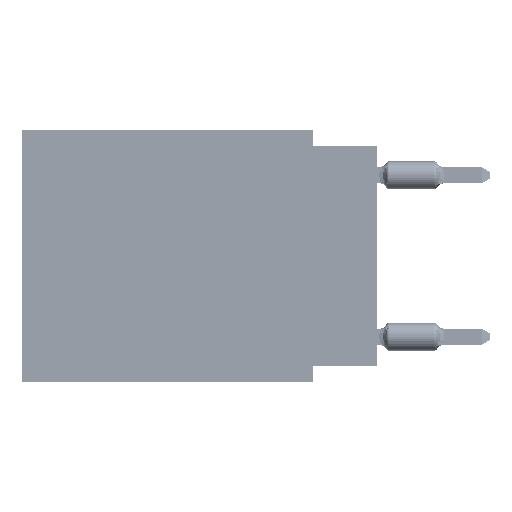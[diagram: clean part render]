
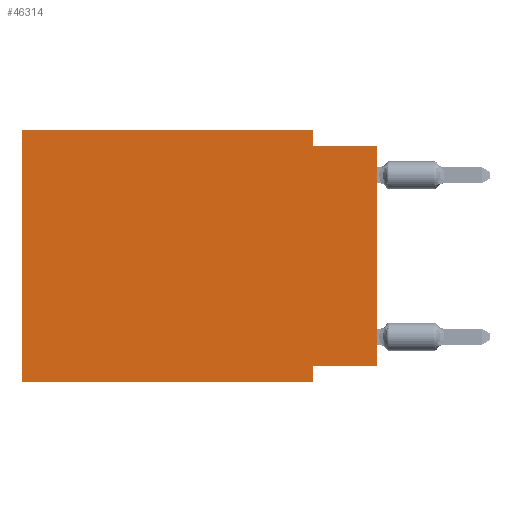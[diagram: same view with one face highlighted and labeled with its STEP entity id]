
A CAD part, left-side view. The second image highlights one B-rep face of the part: STEP entity #46314.
In plain terms, the highlighted planar face has unit normal (-1, 0, 0).
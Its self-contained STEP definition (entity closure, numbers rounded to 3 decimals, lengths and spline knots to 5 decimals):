
#1452 = DIRECTION ( 'NONE',  ( 0., 1., 0. ) ) ;
#3383 = LINE ( 'NONE', #30743, #34249 ) ;
#4033 = LINE ( 'NONE', #73590, #63360 ) ;
#4944 = DIRECTION ( 'NONE',  ( 0., 0., -1. ) ) ;
#5041 = CARTESIAN_POINT ( 'NONE',  ( 0., 0.1, -0.365 ) ) ;
#6688 = VERTEX_POINT ( 'NONE', #30432 ) ;
#10154 = CARTESIAN_POINT ( 'NONE',  ( 0., 0., -0.025 ) ) ;
#11012 = VERTEX_POINT ( 'NONE', #65334 ) ;
#11158 = EDGE_CURVE ( 'NONE', #77506, #37980, #19530, .T. ) ;
#14460 = LINE ( 'NONE', #21627, #53248 ) ;
#15268 = CARTESIAN_POINT ( 'NONE',  ( 0., 0.55, -0.39 ) ) ;
#15789 = EDGE_LOOP ( 'NONE', ( #80450, #38972, #65333, #28414, #53009, #39994, #20164, #63234 ) ) ;
#15989 = DIRECTION ( 'NONE',  ( 0., 0., -1. ) ) ;
#16854 = LINE ( 'NONE', #22697, #59315 ) ;
#19530 = LINE ( 'NONE', #46908, #31091 ) ;
#20164 = ORIENTED_EDGE ( 'NONE', *, *, #22081, .F. ) ;
#21627 = CARTESIAN_POINT ( 'NONE',  ( 0., 0., -0.365 ) ) ;
#22081 = EDGE_CURVE ( 'NONE', #63224, #22983, #4033, .T. ) ;
#22697 = CARTESIAN_POINT ( 'NONE',  ( 0., 0.1, 0. ) ) ;
#22983 = VERTEX_POINT ( 'NONE', #27564 ) ;
#25158 = EDGE_CURVE ( 'NONE', #77506, #22983, #75802, .T. ) ;
#27564 = CARTESIAN_POINT ( 'NONE',  ( 0., 0.1, -0.39 ) ) ;
#28414 = ORIENTED_EDGE ( 'NONE', *, *, #62690, .F. ) ;
#28687 = DIRECTION ( 'NONE',  ( 0., -1., 0. ) ) ;
#30432 = CARTESIAN_POINT ( 'NONE',  ( 0., 0.1, -0.025 ) ) ;
#30743 = CARTESIAN_POINT ( 'NONE',  ( 0., 0.55, 0. ) ) ;
#31091 = VECTOR ( 'NONE', #52775, 39.37008 ) ;
#32036 = CARTESIAN_POINT ( 'NONE',  ( 0., 0., 0. ) ) ;
#32081 = DIRECTION ( 'NONE',  ( 0., -1., 0. ) ) ;
#34249 = VECTOR ( 'NONE', #32081, 39.37008 ) ;
#37980 = VERTEX_POINT ( 'NONE', #38808 ) ;
#38755 = LINE ( 'NONE', #32036, #80571 ) ;
#38808 = CARTESIAN_POINT ( 'NONE',  ( 0., 0.55, 0. ) ) ;
#38972 = ORIENTED_EDGE ( 'NONE', *, *, #40703, .F. ) ;
#39994 = ORIENTED_EDGE ( 'NONE', *, *, #25158, .T. ) ;
#40703 = EDGE_CURVE ( 'NONE', #6688, #11012, #72194, .T. ) ;
#41505 = VERTEX_POINT ( 'NONE', #70709 ) ;
#46314 = ADVANCED_FACE ( 'NONE', ( #53259 ), #80597, .F. ) ;
#46908 = CARTESIAN_POINT ( 'NONE',  ( 0., 0.55, 0. ) ) ;
#48878 = EDGE_CURVE ( 'NONE', #67339, #11012, #38755, .T. ) ;
#48914 = CARTESIAN_POINT ( 'NONE',  ( 0., 0.55, -0.39 ) ) ;
#49573 = VECTOR ( 'NONE', #28687, 39.37008 ) ;
#49673 = DIRECTION ( 'NONE',  ( 0., -1., 0. ) ) ;
#50067 = CARTESIAN_POINT ( 'NONE',  ( 0., 0.55, 0. ) ) ;
#50461 = EDGE_CURVE ( 'NONE', #41505, #6688, #16854, .T. ) ;
#52775 = DIRECTION ( 'NONE',  ( 0., 0., 1. ) ) ;
#53009 = ORIENTED_EDGE ( 'NONE', *, *, #11158, .F. ) ;
#53248 = VECTOR ( 'NONE', #1452, 39.37008 ) ;
#53259 = FACE_OUTER_BOUND ( 'NONE', #15789, .T. ) ;
#59315 = VECTOR ( 'NONE', #15989, 39.37008 ) ;
#59842 = DIRECTION ( 'NONE',  ( 0., 0., 1. ) ) ;
#62690 = EDGE_CURVE ( 'NONE', #37980, #41505, #3383, .T. ) ;
#63224 = VERTEX_POINT ( 'NONE', #5041 ) ;
#63234 = ORIENTED_EDGE ( 'NONE', *, *, #85033, .F. ) ;
#63360 = VECTOR ( 'NONE', #4944, 39.37008 ) ;
#65333 = ORIENTED_EDGE ( 'NONE', *, *, #50461, .F. ) ;
#65334 = CARTESIAN_POINT ( 'NONE',  ( 0., 0., -0.025 ) ) ;
#66723 = CARTESIAN_POINT ( 'NONE',  ( 0., 0., -0.365 ) ) ;
#67339 = VERTEX_POINT ( 'NONE', #66723 ) ;
#69801 = DIRECTION ( 'NONE',  ( 0., 0., -1. ) ) ;
#70487 = AXIS2_PLACEMENT_3D ( 'NONE', #50067, #84125, #69801 ) ;
#70709 = CARTESIAN_POINT ( 'NONE',  ( 0., 0.1, 0. ) ) ;
#72194 = LINE ( 'NONE', #10154, #81476 ) ;
#73590 = CARTESIAN_POINT ( 'NONE',  ( 0., 0.1, -0.39 ) ) ;
#75802 = LINE ( 'NONE', #48914, #49573 ) ;
#77506 = VERTEX_POINT ( 'NONE', #15268 ) ;
#80450 = ORIENTED_EDGE ( 'NONE', *, *, #48878, .T. ) ;
#80571 = VECTOR ( 'NONE', #59842, 39.37008 ) ;
#80597 = PLANE ( 'NONE',  #70487 ) ;
#81476 = VECTOR ( 'NONE', #49673, 39.37008 ) ;
#84125 = DIRECTION ( 'NONE',  ( 1., 0., 0. ) ) ;
#85033 = EDGE_CURVE ( 'NONE', #67339, #63224, #14460, .T. ) ;
